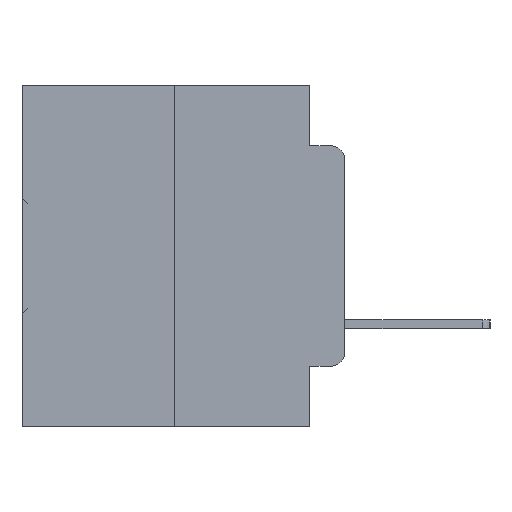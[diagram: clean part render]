
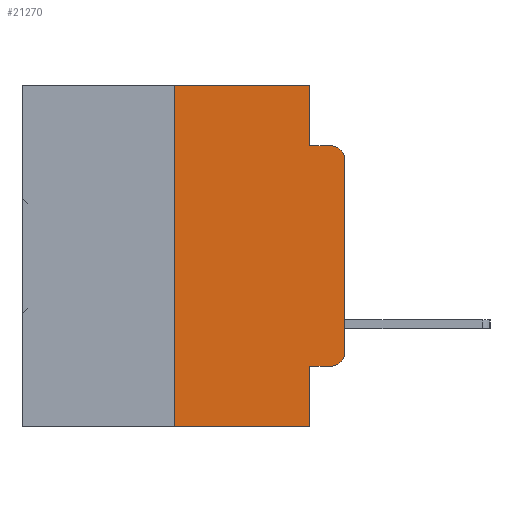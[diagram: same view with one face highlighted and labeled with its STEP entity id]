
A CAD part, left-side view. The second image highlights one B-rep face of the part: STEP entity #21270.
In plain terms, the highlighted planar face has unit normal (-1, 0, 0).
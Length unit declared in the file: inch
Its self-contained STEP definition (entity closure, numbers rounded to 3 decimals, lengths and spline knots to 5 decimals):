
#1030 = CARTESIAN_POINT ( 'NONE',  ( 0., 0., 0. ) ) ;
#1209 = AXIS2_PLACEMENT_3D ( 'NONE', #2660, #21664, #5441 ) ;
#1214 = DIRECTION ( 'NONE',  ( -1., 0., 0. ) ) ;
#1504 = EDGE_CURVE ( 'NONE', #12539, #27343, #29823, .T. ) ;
#1714 = DIRECTION ( 'NONE',  ( 0., 0., 1. ) ) ;
#1779 = VECTOR ( 'NONE', #26129, 39.37008 ) ;
#2087 = DIRECTION ( 'NONE',  ( 0., 0., -1. ) ) ;
#2437 = VERTEX_POINT ( 'NONE', #26520 ) ;
#2660 = CARTESIAN_POINT ( 'NONE',  ( 0., 0.02, -0.3915 ) ) ;
#2758 = CARTESIAN_POINT ( 'NONE',  ( 0., 0.051, -0.5 ) ) ;
#2825 = CARTESIAN_POINT ( 'NONE',  ( 0., 0.473, 0. ) ) ;
#2842 = EDGE_CURVE ( 'NONE', #16043, #3018, #14751, .T. ) ;
#3018 = VERTEX_POINT ( 'NONE', #12841 ) ;
#3540 = VERTEX_POINT ( 'NONE', #15163 ) ;
#4318 = PLANE ( 'NONE',  #7653 ) ;
#4338 = FACE_OUTER_BOUND ( 'NONE', #25629, .T. ) ;
#4585 = CARTESIAN_POINT ( 'NONE',  ( 0., 0.051, -0.0885 ) ) ;
#4896 = LINE ( 'NONE', #16128, #26370 ) ;
#4899 = LINE ( 'NONE', #20200, #18490 ) ;
#5377 = EDGE_CURVE ( 'NONE', #2437, #12539, #27474, .T. ) ;
#5441 = DIRECTION ( 'NONE',  ( 0., 0., -1. ) ) ;
#6532 = EDGE_CURVE ( 'NONE', #34737, #16043, #31129, .T. ) ;
#6602 = ORIENTED_EDGE ( 'NONE', *, *, #22368, .T. ) ;
#7062 = CARTESIAN_POINT ( 'NONE',  ( 0., 0.473, 0. ) ) ;
#7653 = AXIS2_PLACEMENT_3D ( 'NONE', #7062, #12575, #31167 ) ;
#8055 = VERTEX_POINT ( 'NONE', #2758 ) ;
#9863 = VECTOR ( 'NONE', #12101, 39.37008 ) ;
#12101 = DIRECTION ( 'NONE',  ( 0., 0., 1. ) ) ;
#12539 = VERTEX_POINT ( 'NONE', #19264 ) ;
#12575 = DIRECTION ( 'NONE',  ( 1., 0., 0. ) ) ;
#12841 = CARTESIAN_POINT ( 'NONE',  ( 0., 0.02, -0.0885 ) ) ;
#14611 = DIRECTION ( 'NONE',  ( 0., -1., 0. ) ) ;
#14751 = CIRCLE ( 'NONE', #21542, 0.02 ) ;
#15163 = CARTESIAN_POINT ( 'NONE',  ( 0., 0.051, -0.4115 ) ) ;
#15720 = CARTESIAN_POINT ( 'NONE',  ( 0., 0.051, 0. ) ) ;
#16043 = VERTEX_POINT ( 'NONE', #34360 ) ;
#16128 = CARTESIAN_POINT ( 'NONE',  ( 0., 0.051, 0. ) ) ;
#17005 = CARTESIAN_POINT ( 'NONE',  ( 0., 0.051, 0. ) ) ;
#17018 = DIRECTION ( 'NONE',  ( 0., -1., 0. ) ) ;
#17035 = VECTOR ( 'NONE', #14611, 39.37008 ) ;
#17579 = CARTESIAN_POINT ( 'NONE',  ( 0., 0.02, -0.1085 ) ) ;
#18490 = VECTOR ( 'NONE', #22827, 39.37008 ) ;
#18550 = CARTESIAN_POINT ( 'NONE',  ( 0., 0., -0.3915 ) ) ;
#18769 = VECTOR ( 'NONE', #1714, 39.37008 ) ;
#19264 = CARTESIAN_POINT ( 'NONE',  ( 0., 0.25, 0. ) ) ;
#20200 = CARTESIAN_POINT ( 'NONE',  ( 0., 0.051, -0.4115 ) ) ;
#20287 = DIRECTION ( 'NONE',  ( 0., 0., -1. ) ) ;
#21270 = ADVANCED_FACE ( 'NONE', ( #4338 ), #4318, .F. ) ;
#21381 = ORIENTED_EDGE ( 'NONE', *, *, #22620, .T. ) ;
#21542 = AXIS2_PLACEMENT_3D ( 'NONE', #17579, #1214, #20287 ) ;
#21664 = DIRECTION ( 'NONE',  ( -1., 0., 0. ) ) ;
#22024 = VECTOR ( 'NONE', #17018, 39.37008 ) ;
#22319 = CARTESIAN_POINT ( 'NONE',  ( 0., 0.02, -0.4115 ) ) ;
#22368 = EDGE_CURVE ( 'NONE', #28710, #34737, #24509, .T. ) ;
#22620 = EDGE_CURVE ( 'NONE', #2437, #8055, #31886, .T. ) ;
#22827 = DIRECTION ( 'NONE',  ( 0., -1., 0. ) ) ;
#24509 = CIRCLE ( 'NONE', #1209, 0.02 ) ;
#24989 = ORIENTED_EDGE ( 'NONE', *, *, #2842, .T. ) ;
#25078 = ORIENTED_EDGE ( 'NONE', *, *, #1504, .F. ) ;
#25231 = EDGE_CURVE ( 'NONE', #27343, #33281, #29704, .T. ) ;
#25629 = EDGE_LOOP ( 'NONE', ( #28754, #24989, #26791, #27428, #25078, #26732, #21381, #31656, #27191, #6602 ) ) ;
#26129 = DIRECTION ( 'NONE',  ( 0., -1., 0. ) ) ;
#26370 = VECTOR ( 'NONE', #26800, 39.37008 ) ;
#26520 = CARTESIAN_POINT ( 'NONE',  ( 0., 0.25, -0.5 ) ) ;
#26732 = ORIENTED_EDGE ( 'NONE', *, *, #5377, .F. ) ;
#26791 = ORIENTED_EDGE ( 'NONE', *, *, #34003, .F. ) ;
#26800 = DIRECTION ( 'NONE',  ( 0., 0., -1. ) ) ;
#27191 = ORIENTED_EDGE ( 'NONE', *, *, #29414, .T. ) ;
#27343 = VERTEX_POINT ( 'NONE', #17005 ) ;
#27428 = ORIENTED_EDGE ( 'NONE', *, *, #25231, .F. ) ;
#27474 = LINE ( 'NONE', #31208, #18769 ) ;
#27874 = CARTESIAN_POINT ( 'NONE',  ( 0., 0.473, -0.5 ) ) ;
#28710 = VERTEX_POINT ( 'NONE', #22319 ) ;
#28754 = ORIENTED_EDGE ( 'NONE', *, *, #6532, .T. ) ;
#28896 = VECTOR ( 'NONE', #2087, 39.37008 ) ;
#29414 = EDGE_CURVE ( 'NONE', #3540, #28710, #4899, .T. ) ;
#29704 = LINE ( 'NONE', #15720, #28896 ) ;
#29823 = LINE ( 'NONE', #2825, #22024 ) ;
#30394 = LINE ( 'NONE', #4585, #1779 ) ;
#30884 = CARTESIAN_POINT ( 'NONE',  ( 0., 0.051, -0.0885 ) ) ;
#31129 = LINE ( 'NONE', #1030, #9863 ) ;
#31167 = DIRECTION ( 'NONE',  ( 0., 0., -1. ) ) ;
#31208 = CARTESIAN_POINT ( 'NONE',  ( 0., 0.25, 0. ) ) ;
#31656 = ORIENTED_EDGE ( 'NONE', *, *, #32908, .F. ) ;
#31886 = LINE ( 'NONE', #27874, #17035 ) ;
#32908 = EDGE_CURVE ( 'NONE', #3540, #8055, #4896, .T. ) ;
#33281 = VERTEX_POINT ( 'NONE', #30884 ) ;
#34003 = EDGE_CURVE ( 'NONE', #33281, #3018, #30394, .T. ) ;
#34360 = CARTESIAN_POINT ( 'NONE',  ( 0., 0., -0.1085 ) ) ;
#34737 = VERTEX_POINT ( 'NONE', #18550 ) ;
